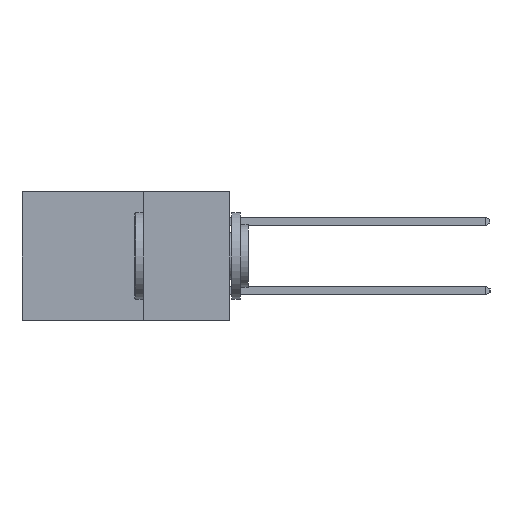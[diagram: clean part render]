
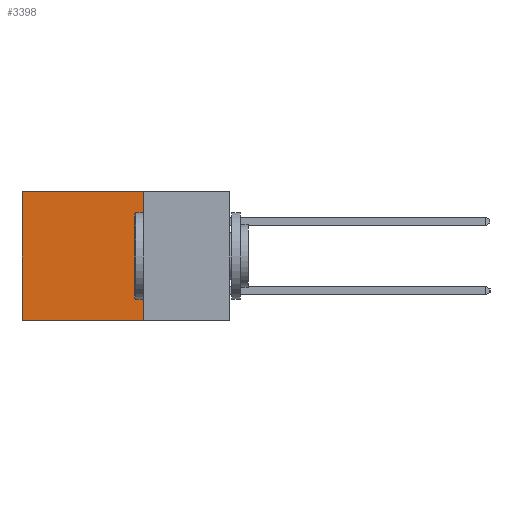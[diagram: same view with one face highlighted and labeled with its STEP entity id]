
A CAD part, left-side view. The second image highlights one B-rep face of the part: STEP entity #3398.
In plain terms, the highlighted planar face has unit normal (-1, 0, 0).
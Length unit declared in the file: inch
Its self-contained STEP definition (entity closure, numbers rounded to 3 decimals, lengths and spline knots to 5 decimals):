
#1224 = LINE ( 'NONE', #10596, #4178 ) ;
#2424 = EDGE_CURVE ( 'NONE', #3568, #4575, #6633, .T. ) ;
#2499 = ORIENTED_EDGE ( 'NONE', *, *, #2564, .F. ) ;
#2564 = EDGE_CURVE ( 'NONE', #4899, #6929, #1224, .T. ) ;
#3398 = ADVANCED_FACE ( 'NONE', ( #8642 ), #11483, .F. ) ;
#3414 = CARTESIAN_POINT ( 'NONE',  ( 0.2615, 0.6, -0.37 ) ) ;
#3568 = VERTEX_POINT ( 'NONE', #4821 ) ;
#3581 = EDGE_CURVE ( 'NONE', #6929, #4575, #9166, .T. ) ;
#3646 = VECTOR ( 'NONE', #8584, 39.37008 ) ;
#4178 = VECTOR ( 'NONE', #10593, 39.37008 ) ;
#4202 = DIRECTION ( 'NONE',  ( 0., 1., 0. ) ) ;
#4389 = CARTESIAN_POINT ( 'NONE',  ( 0.2615, 0.25, 0. ) ) ;
#4575 = VERTEX_POINT ( 'NONE', #3414 ) ;
#4821 = CARTESIAN_POINT ( 'NONE',  ( 0.2615, 0.6, 0. ) ) ;
#4899 = VERTEX_POINT ( 'NONE', #4389 ) ;
#5124 = CARTESIAN_POINT ( 'NONE',  ( 0.2615, 0.25, -0.37 ) ) ;
#6633 = LINE ( 'NONE', #13126, #11964 ) ;
#6929 = VERTEX_POINT ( 'NONE', #10043 ) ;
#6975 = CARTESIAN_POINT ( 'NONE',  ( 0.2615, 0.25, -0.37 ) ) ;
#7159 = ORIENTED_EDGE ( 'NONE', *, *, #12410, .T. ) ;
#7464 = EDGE_LOOP ( 'NONE', ( #12539, #8044, #2499, #7159 ) ) ;
#8044 = ORIENTED_EDGE ( 'NONE', *, *, #3581, .F. ) ;
#8584 = DIRECTION ( 'NONE',  ( 0., 1., 0. ) ) ;
#8642 = FACE_OUTER_BOUND ( 'NONE', #7464, .T. ) ;
#9166 = LINE ( 'NONE', #5124, #3646 ) ;
#9850 = LINE ( 'NONE', #10748, #12875 ) ;
#10043 = CARTESIAN_POINT ( 'NONE',  ( 0.2615, 0.25, -0.37 ) ) ;
#10593 = DIRECTION ( 'NONE',  ( 0., 0., -1. ) ) ;
#10596 = CARTESIAN_POINT ( 'NONE',  ( 0.2615, 0.25, -0.37 ) ) ;
#10748 = CARTESIAN_POINT ( 'NONE',  ( 0.2615, 0.25, 0. ) ) ;
#10789 = AXIS2_PLACEMENT_3D ( 'NONE', #6975, #13458, #13432 ) ;
#11483 = PLANE ( 'NONE',  #10789 ) ;
#11964 = VECTOR ( 'NONE', #13269, 39.37008 ) ;
#12410 = EDGE_CURVE ( 'NONE', #4899, #3568, #9850, .T. ) ;
#12539 = ORIENTED_EDGE ( 'NONE', *, *, #2424, .T. ) ;
#12875 = VECTOR ( 'NONE', #4202, 39.37008 ) ;
#13126 = CARTESIAN_POINT ( 'NONE',  ( 0.2615, 0.6, -0.37 ) ) ;
#13269 = DIRECTION ( 'NONE',  ( 0., 0., -1. ) ) ;
#13432 = DIRECTION ( 'NONE',  ( 0., 0., -1. ) ) ;
#13458 = DIRECTION ( 'NONE',  ( 1., 0., 0. ) ) ;
